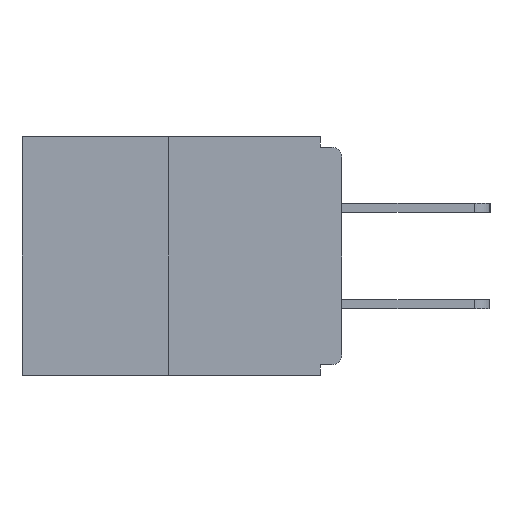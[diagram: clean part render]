
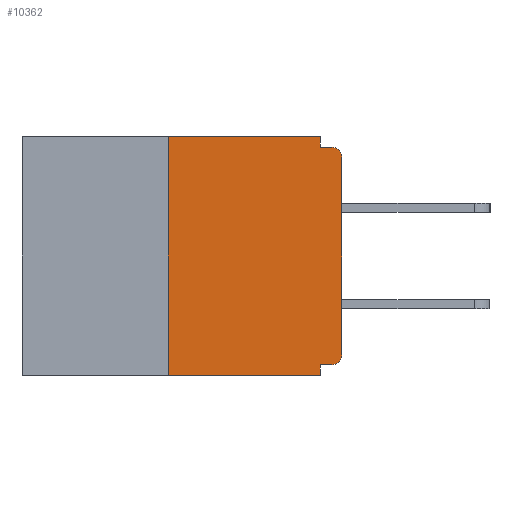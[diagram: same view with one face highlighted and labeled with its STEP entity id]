
A CAD part, left-side view. The second image highlights one B-rep face of the part: STEP entity #10362.
In plain terms, the highlighted planar face has unit normal (-1, 0, 0).
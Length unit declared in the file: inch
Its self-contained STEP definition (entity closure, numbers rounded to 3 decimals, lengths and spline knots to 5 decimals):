
#26 = CARTESIAN_POINT ( 'NONE',  ( 0., 0.46, -0.343 ) ) ;
#306 = CARTESIAN_POINT ( 'NONE',  ( 0., 0.031, -0.015 ) ) ;
#416 = VERTEX_POINT ( 'NONE', #3997 ) ;
#918 = CARTESIAN_POINT ( 'NONE',  ( 0., 0., -0.328 ) ) ;
#968 = CARTESIAN_POINT ( 'NONE',  ( 0., 0.25, 0. ) ) ;
#1142 = ORIENTED_EDGE ( 'NONE', *, *, #16402, .T. ) ;
#1176 = VERTEX_POINT ( 'NONE', #4521 ) ;
#1188 = LINE ( 'NONE', #13968, #10047 ) ;
#1373 = ORIENTED_EDGE ( 'NONE', *, *, #13102, .F. ) ;
#1451 = CARTESIAN_POINT ( 'NONE',  ( 0., 0., -0.313 ) ) ;
#1973 = CARTESIAN_POINT ( 'NONE',  ( 0., 0., -0.015 ) ) ;
#2386 = AXIS2_PLACEMENT_3D ( 'NONE', #15434, #5168, #6889 ) ;
#2580 = ORIENTED_EDGE ( 'NONE', *, *, #4196, .T. ) ;
#2754 = VECTOR ( 'NONE', #20711, 39.37008 ) ;
#2903 = VECTOR ( 'NONE', #7696, 39.37008 ) ;
#3446 = PLANE ( 'NONE',  #2386 ) ;
#3997 = CARTESIAN_POINT ( 'NONE',  ( 0., 0., -0.03 ) ) ;
#4196 = EDGE_CURVE ( 'NONE', #16654, #416, #20968, .T. ) ;
#4521 = CARTESIAN_POINT ( 'NONE',  ( 0., 0.015, -0.328 ) ) ;
#4773 = EDGE_CURVE ( 'NONE', #1176, #16654, #9839, .T. ) ;
#4905 = DIRECTION ( 'NONE',  ( 0., 0., -1. ) ) ;
#5168 = DIRECTION ( 'NONE',  ( 1., 0., 0. ) ) ;
#5414 = DIRECTION ( 'NONE',  ( 0., 0., -1. ) ) ;
#5787 = EDGE_CURVE ( 'NONE', #416, #21316, #11659, .T. ) ;
#6429 = CARTESIAN_POINT ( 'NONE',  ( 0., 0.031, -0.343 ) ) ;
#6829 = EDGE_CURVE ( 'NONE', #12746, #12596, #21350, .T. ) ;
#6889 = DIRECTION ( 'NONE',  ( 0., 0., -1. ) ) ;
#7341 = AXIS2_PLACEMENT_3D ( 'NONE', #10813, #13940, #5414 ) ;
#7696 = DIRECTION ( 'NONE',  ( 0., 1., 0. ) ) ;
#7735 = VECTOR ( 'NONE', #11242, 39.37008 ) ;
#8424 = DIRECTION ( 'NONE',  ( -1., 0., 0. ) ) ;
#8568 = LINE ( 'NONE', #918, #2903 ) ;
#8652 = LINE ( 'NONE', #21901, #9424 ) ;
#8849 = CARTESIAN_POINT ( 'NONE',  ( 0., 0.031, -0.328 ) ) ;
#9424 = VECTOR ( 'NONE', #4905, 39.37008 ) ;
#9839 = CIRCLE ( 'NONE', #7341, 0.015 ) ;
#10008 = CARTESIAN_POINT ( 'NONE',  ( 0., 0.015, -0.015 ) ) ;
#10047 = VECTOR ( 'NONE', #14471, 39.37008 ) ;
#10126 = DIRECTION ( 'NONE',  ( 0., 0., -1. ) ) ;
#10362 = ADVANCED_FACE ( 'NONE', ( #12905 ), #3446, .F. ) ;
#10669 = AXIS2_PLACEMENT_3D ( 'NONE', #18644, #8424, #10126 ) ;
#10787 = EDGE_CURVE ( 'NONE', #14802, #17930, #8652, .T. ) ;
#10803 = ORIENTED_EDGE ( 'NONE', *, *, #15092, .F. ) ;
#10813 = CARTESIAN_POINT ( 'NONE',  ( 0., 0.015, -0.313 ) ) ;
#11180 = ORIENTED_EDGE ( 'NONE', *, *, #5787, .T. ) ;
#11242 = DIRECTION ( 'NONE',  ( 0., 0., 1. ) ) ;
#11659 = CIRCLE ( 'NONE', #10669, 0.015 ) ;
#12417 = LINE ( 'NONE', #1973, #2754 ) ;
#12552 = CARTESIAN_POINT ( 'NONE',  ( 0., 0.25, -0.343 ) ) ;
#12596 = VERTEX_POINT ( 'NONE', #306 ) ;
#12746 = VERTEX_POINT ( 'NONE', #15816 ) ;
#12905 = FACE_OUTER_BOUND ( 'NONE', #15206, .T. ) ;
#13091 = VECTOR ( 'NONE', #15077, 39.37008 ) ;
#13102 = EDGE_CURVE ( 'NONE', #1176, #14802, #8568, .T. ) ;
#13206 = VERTEX_POINT ( 'NONE', #13429 ) ;
#13351 = CARTESIAN_POINT ( 'NONE',  ( 0., 0., 0. ) ) ;
#13429 = CARTESIAN_POINT ( 'NONE',  ( 0., 0.25, 0. ) ) ;
#13551 = ORIENTED_EDGE ( 'NONE', *, *, #16148, .F. ) ;
#13940 = DIRECTION ( 'NONE',  ( -1., 0., 0. ) ) ;
#13968 = CARTESIAN_POINT ( 'NONE',  ( 0., 0.46, 0. ) ) ;
#14471 = DIRECTION ( 'NONE',  ( 0., -1., 0. ) ) ;
#14802 = VERTEX_POINT ( 'NONE', #8849 ) ;
#15077 = DIRECTION ( 'NONE',  ( 0., 0., 1. ) ) ;
#15092 = EDGE_CURVE ( 'NONE', #13206, #12746, #1188, .T. ) ;
#15206 = EDGE_LOOP ( 'NONE', ( #10803, #16795, #1142, #19226, #1373, #17054, #2580, #11180, #13551, #21687 ) ) ;
#15434 = CARTESIAN_POINT ( 'NONE',  ( 0., 0.46, 0. ) ) ;
#15816 = CARTESIAN_POINT ( 'NONE',  ( 0., 0.031, 0. ) ) ;
#16148 = EDGE_CURVE ( 'NONE', #12596, #21316, #12417, .T. ) ;
#16358 = DIRECTION ( 'NONE',  ( 0., 0., -1. ) ) ;
#16402 = EDGE_CURVE ( 'NONE', #18477, #17930, #18826, .T. ) ;
#16654 = VERTEX_POINT ( 'NONE', #1451 ) ;
#16795 = ORIENTED_EDGE ( 'NONE', *, *, #16842, .F. ) ;
#16842 = EDGE_CURVE ( 'NONE', #18477, #13206, #19258, .T. ) ;
#17054 = ORIENTED_EDGE ( 'NONE', *, *, #4773, .T. ) ;
#17930 = VERTEX_POINT ( 'NONE', #6429 ) ;
#18477 = VERTEX_POINT ( 'NONE', #12552 ) ;
#18644 = CARTESIAN_POINT ( 'NONE',  ( 0., 0.015, -0.03 ) ) ;
#18826 = LINE ( 'NONE', #26, #19367 ) ;
#19226 = ORIENTED_EDGE ( 'NONE', *, *, #10787, .F. ) ;
#19258 = LINE ( 'NONE', #968, #7735 ) ;
#19367 = VECTOR ( 'NONE', #20301, 39.37008 ) ;
#19974 = CARTESIAN_POINT ( 'NONE',  ( 0., 0.031, 0. ) ) ;
#20301 = DIRECTION ( 'NONE',  ( 0., -1., 0. ) ) ;
#20711 = DIRECTION ( 'NONE',  ( 0., -1., 0. ) ) ;
#20968 = LINE ( 'NONE', #13351, #13091 ) ;
#21053 = VECTOR ( 'NONE', #16358, 39.37008 ) ;
#21316 = VERTEX_POINT ( 'NONE', #10008 ) ;
#21350 = LINE ( 'NONE', #19974, #21053 ) ;
#21687 = ORIENTED_EDGE ( 'NONE', *, *, #6829, .F. ) ;
#21901 = CARTESIAN_POINT ( 'NONE',  ( 0., 0.031, -0.343 ) ) ;
